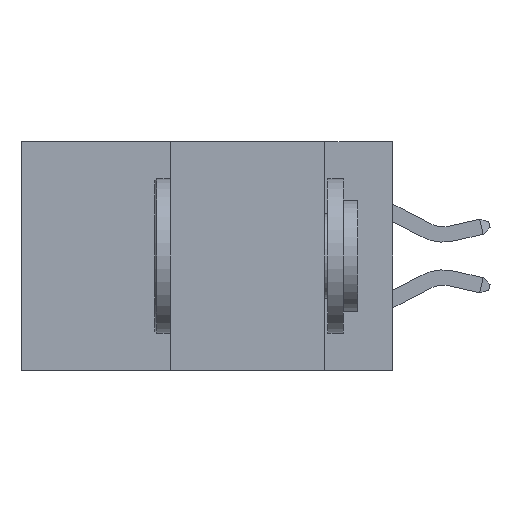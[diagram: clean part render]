
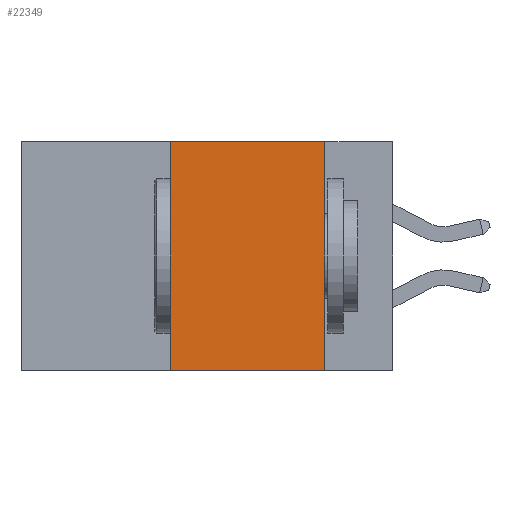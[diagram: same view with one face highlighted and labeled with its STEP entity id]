
A CAD part, left-side view. The second image highlights one B-rep face of the part: STEP entity #22349.
In plain terms, the highlighted planar face has unit normal (-1, 0, 0).
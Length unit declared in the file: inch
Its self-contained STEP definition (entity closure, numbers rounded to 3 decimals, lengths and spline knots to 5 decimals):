
#50 = CARTESIAN_POINT ( 'NONE',  ( 0., 0.6, -0.37 ) ) ;
#589 = LINE ( 'NONE', #7648, #16231 ) ;
#876 = ORIENTED_EDGE ( 'NONE', *, *, #6831, .F. ) ;
#1409 = EDGE_LOOP ( 'NONE', ( #876, #7834, #13299, #23059 ) ) ;
#2683 = CARTESIAN_POINT ( 'NONE',  ( 0., 0.36, -0.37 ) ) ;
#2784 = VERTEX_POINT ( 'NONE', #7238 ) ;
#4271 = EDGE_CURVE ( 'NONE', #15247, #5523, #589, .T. ) ;
#5373 = VECTOR ( 'NONE', #7519, 39.37008 ) ;
#5523 = VERTEX_POINT ( 'NONE', #20631 ) ;
#5608 = CARTESIAN_POINT ( 'NONE',  ( 0., 0.11, 0. ) ) ;
#6831 = EDGE_CURVE ( 'NONE', #2784, #17493, #20159, .T. ) ;
#7225 = DIRECTION ( 'NONE',  ( 0., -1., 0. ) ) ;
#7238 = CARTESIAN_POINT ( 'NONE',  ( 0., 0.11, 0. ) ) ;
#7519 = DIRECTION ( 'NONE',  ( 0., 0., -1. ) ) ;
#7648 = CARTESIAN_POINT ( 'NONE',  ( 0., 0.36, 0. ) ) ;
#7683 = DIRECTION ( 'NONE',  ( 0., 0., 1. ) ) ;
#7834 = ORIENTED_EDGE ( 'NONE', *, *, #16105, .F. ) ;
#10278 = LINE ( 'NONE', #23773, #10851 ) ;
#10292 = CARTESIAN_POINT ( 'NONE',  ( 0., 0.6, 0. ) ) ;
#10851 = VECTOR ( 'NONE', #7225, 39.37008 ) ;
#12125 = DIRECTION ( 'NONE',  ( 0., 0., -1. ) ) ;
#13299 = ORIENTED_EDGE ( 'NONE', *, *, #4271, .F. ) ;
#13911 = PLANE ( 'NONE',  #20563 ) ;
#15106 = VECTOR ( 'NONE', #15243, 39.37008 ) ;
#15243 = DIRECTION ( 'NONE',  ( 0., -1., 0. ) ) ;
#15247 = VERTEX_POINT ( 'NONE', #2683 ) ;
#16105 = EDGE_CURVE ( 'NONE', #5523, #2784, #10278, .T. ) ;
#16231 = VECTOR ( 'NONE', #7683, 39.37008 ) ;
#17493 = VERTEX_POINT ( 'NONE', #22079 ) ;
#20010 = LINE ( 'NONE', #50, #15106 ) ;
#20159 = LINE ( 'NONE', #5608, #5373 ) ;
#20563 = AXIS2_PLACEMENT_3D ( 'NONE', #10292, #23120, #12125 ) ;
#20631 = CARTESIAN_POINT ( 'NONE',  ( 0., 0.36, 0. ) ) ;
#21760 = FACE_OUTER_BOUND ( 'NONE', #1409, .T. ) ;
#22079 = CARTESIAN_POINT ( 'NONE',  ( 0., 0.11, -0.37 ) ) ;
#22349 = ADVANCED_FACE ( 'NONE', ( #21760 ), #13911, .F. ) ;
#23059 = ORIENTED_EDGE ( 'NONE', *, *, #23313, .T. ) ;
#23120 = DIRECTION ( 'NONE',  ( 1., 0., 0. ) ) ;
#23313 = EDGE_CURVE ( 'NONE', #15247, #17493, #20010, .T. ) ;
#23773 = CARTESIAN_POINT ( 'NONE',  ( 0., 0.6, 0. ) ) ;
